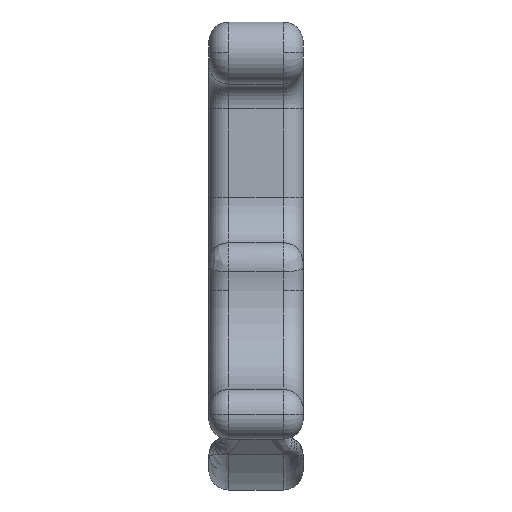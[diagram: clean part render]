
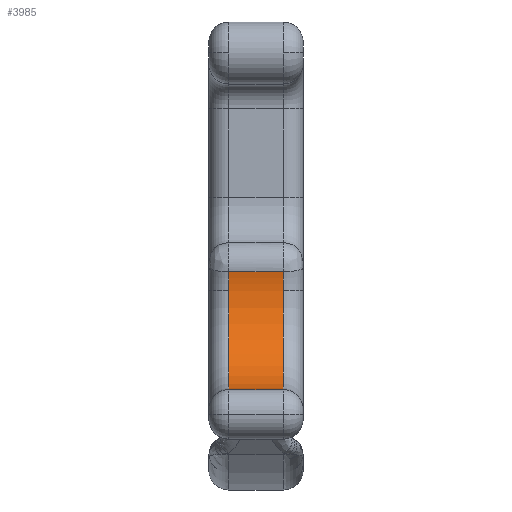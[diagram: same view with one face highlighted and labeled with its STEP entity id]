
A CAD part, top view. The second image highlights one B-rep face of the part: STEP entity #3985.
In plain terms, the highlighted cylindrical face has radius 10 mm (diameter 20 mm), a partial arc.
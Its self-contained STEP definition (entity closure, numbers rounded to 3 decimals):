
#35 = LINE ( 'NONE', #3484, #1410 ) ;
#146 = CARTESIAN_POINT ( 'NONE',  ( 3.833, 6.902, 35.182 ) ) ;
#231 = DIRECTION ( 'NONE',  ( 0., 0., -1. ) ) ;
#341 = DIRECTION ( 'NONE',  ( 0., 0., 1. ) ) ;
#414 = CARTESIAN_POINT ( 'NONE',  ( 7.5, 6.902, 35.182 ) ) ;
#434 = CARTESIAN_POINT ( 'NONE',  ( 7.5, 5., 45. ) ) ;
#538 = VERTEX_POINT ( 'NONE', #2452 ) ;
#686 = CARTESIAN_POINT ( 'NONE',  ( 9.5, 5., 45. ) ) ;
#753 = CARTESIAN_POINT ( 'NONE',  ( 7.5, 6.902, 35.182 ) ) ;
#784 = DIRECTION ( 'NONE',  ( 0., 0., -1. ) ) ;
#865 = ORIENTED_EDGE ( 'NONE', *, *, #1326, .T. ) ;
#1000 = ORIENTED_EDGE ( 'NONE', *, *, #2769, .T. ) ;
#1035 = DIRECTION ( 'NONE',  ( -1., 0., 0. ) ) ;
#1037 = CARTESIAN_POINT ( 'NONE',  ( 2., -5., 45. ) ) ;
#1326 = EDGE_CURVE ( 'NONE', #3020, #3002, #3058, .T. ) ;
#1410 = VECTOR ( 'NONE', #3493, 1000. ) ;
#1452 = AXIS2_PLACEMENT_3D ( 'NONE', #434, #2812, #784 ) ;
#1532 = CIRCLE ( 'NONE', #4001, 10. ) ;
#1622 = EDGE_CURVE ( 'NONE', #2375, #1744, #1532, .T. ) ;
#1638 = ORIENTED_EDGE ( 'NONE', *, *, #3158, .F. ) ;
#1650 = EDGE_LOOP ( 'NONE', ( #865, #1000, #3789, #1638, #4078, #2574 ) ) ;
#1667 = DIRECTION ( 'NONE',  ( -1., 0., 0. ) ) ;
#1724 = AXIS2_PLACEMENT_3D ( 'NONE', #4245, #2268, #231 ) ;
#1744 = VERTEX_POINT ( 'NONE', #2168 ) ;
#1748 = AXIS2_PLACEMENT_3D ( 'NONE', #686, #1035, #341 ) ;
#1775 = CARTESIAN_POINT ( 'NONE',  ( 7.5, 5., 45. ) ) ;
#1786 = CARTESIAN_POINT ( 'NONE',  ( 5.667, 6.902, 35.182 ) ) ;
#1862 = FACE_OUTER_BOUND ( 'NONE', #1650, .T. ) ;
#2108 = DIRECTION ( 'NONE',  ( 0., 0., -1. ) ) ;
#2149 = VERTEX_POINT ( 'NONE', #1037 ) ;
#2168 = CARTESIAN_POINT ( 'NONE',  ( 7.5, 5., 35. ) ) ;
#2268 = DIRECTION ( 'NONE',  ( -1., 0., 0. ) ) ;
#2375 = VERTEX_POINT ( 'NONE', #2611 ) ;
#2434 = EDGE_CURVE ( 'NONE', #538, #2149, #3555, .T. ) ;
#2445 = CARTESIAN_POINT ( 'NONE',  ( 2., 6.902, 35.182 ) ) ;
#2452 = CARTESIAN_POINT ( 'NONE',  ( 2., 5., 35. ) ) ;
#2507 = CARTESIAN_POINT ( 'NONE',  ( 2., 6.902, 35.182 ) ) ;
#2574 = ORIENTED_EDGE ( 'NONE', *, *, #3463, .T. ) ;
#2611 = CARTESIAN_POINT ( 'NONE',  ( 7.5, -5., 45. ) ) ;
#2769 = EDGE_CURVE ( 'NONE', #3002, #538, #3052, .T. ) ;
#2812 = DIRECTION ( 'NONE',  ( 1., 0., 0. ) ) ;
#3002 = VERTEX_POINT ( 'NONE', #2445 ) ;
#3020 = VERTEX_POINT ( 'NONE', #414 ) ;
#3052 = CIRCLE ( 'NONE', #1724, 10. ) ;
#3058 = B_SPLINE_CURVE_WITH_KNOTS ( 'NONE', 3,
 ( #753, #1786, #146, #2507 ),
 .UNSPECIFIED., .F., .F.,
 ( 4, 4 ),
 ( 0.211, 0.789 ),
 .UNSPECIFIED. ) ;
#3158 = EDGE_CURVE ( 'NONE', #2375, #2149, #35, .T. ) ;
#3463 = EDGE_CURVE ( 'NONE', #1744, #3020, #4109, .T. ) ;
#3484 = CARTESIAN_POINT ( 'NONE',  ( 9.5, -5., 45. ) ) ;
#3493 = DIRECTION ( 'NONE',  ( -1., 0., 0. ) ) ;
#3555 = CIRCLE ( 'NONE', #4105, 10. ) ;
#3653 = CARTESIAN_POINT ( 'NONE',  ( 2., 5., 45. ) ) ;
#3789 = ORIENTED_EDGE ( 'NONE', *, *, #2434, .T. ) ;
#3985 = ADVANCED_FACE ( 'NONE', ( #1862 ), #4314, .F. ) ;
#3988 = DIRECTION ( 'NONE',  ( 0., 0., -1. ) ) ;
#4001 = AXIS2_PLACEMENT_3D ( 'NONE', #1775, #4096, #2108 ) ;
#4078 = ORIENTED_EDGE ( 'NONE', *, *, #1622, .T. ) ;
#4096 = DIRECTION ( 'NONE',  ( 1., 0., 0. ) ) ;
#4105 = AXIS2_PLACEMENT_3D ( 'NONE', #3653, #1667, #3988 ) ;
#4109 = CIRCLE ( 'NONE', #1452, 10. ) ;
#4245 = CARTESIAN_POINT ( 'NONE',  ( 2., 5., 45. ) ) ;
#4314 = CYLINDRICAL_SURFACE ( 'NONE', #1748, 10. ) ;
